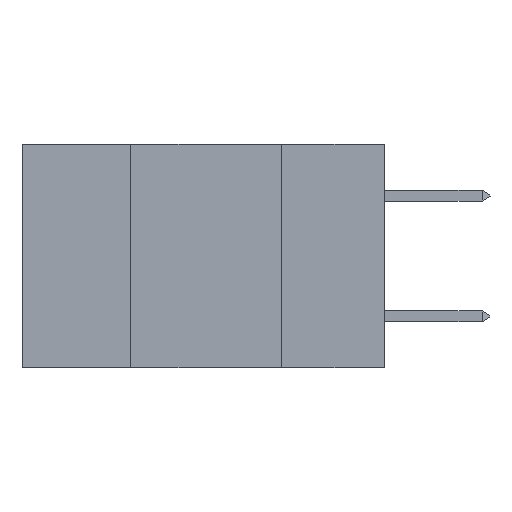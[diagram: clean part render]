
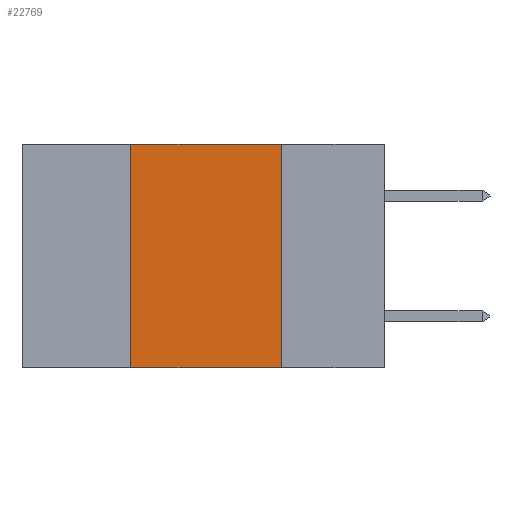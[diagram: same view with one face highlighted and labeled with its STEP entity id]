
A CAD part, left-side view. The second image highlights one B-rep face of the part: STEP entity #22769.
In plain terms, the highlighted planar face has unit normal (-1, 0, 0).
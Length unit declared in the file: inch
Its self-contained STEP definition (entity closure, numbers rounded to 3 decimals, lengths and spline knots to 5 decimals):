
#1746 = ORIENTED_EDGE ( 'NONE', *, *, #6668, .F. ) ;
#2433 = CARTESIAN_POINT ( 'NONE',  ( 0., 0.42, 0. ) ) ;
#4499 = CARTESIAN_POINT ( 'NONE',  ( 0., 0.17, 0. ) ) ;
#6262 = CARTESIAN_POINT ( 'NONE',  ( 0., 0.17, 0. ) ) ;
#6668 = EDGE_CURVE ( 'NONE', #8438, #32411, #27385, .T. ) ;
#8362 = CARTESIAN_POINT ( 'NONE',  ( 0., 0.42, 0. ) ) ;
#8438 = VERTEX_POINT ( 'NONE', #2433 ) ;
#10144 = AXIS2_PLACEMENT_3D ( 'NONE', #35206, #35842, #25653 ) ;
#10730 = CARTESIAN_POINT ( 'NONE',  ( 0., 0.6, 0. ) ) ;
#12917 = ORIENTED_EDGE ( 'NONE', *, *, #26547, .F. ) ;
#15918 = FACE_OUTER_BOUND ( 'NONE', #27540, .T. ) ;
#19678 = LINE ( 'NONE', #6262, #37591 ) ;
#22769 = ADVANCED_FACE ( 'NONE', ( #15918 ), #42349, .F. ) ;
#23365 = VERTEX_POINT ( 'NONE', #29712 ) ;
#23923 = DIRECTION ( 'NONE',  ( 0., -1., 0. ) ) ;
#25653 = DIRECTION ( 'NONE',  ( 0., 0., -1. ) ) ;
#26547 = EDGE_CURVE ( 'NONE', #32411, #34997, #19678, .T. ) ;
#27385 = LINE ( 'NONE', #10730, #27852 ) ;
#27500 = VECTOR ( 'NONE', #41761, 39.37008 ) ;
#27540 = EDGE_LOOP ( 'NONE', ( #12917, #1746, #29695, #37684 ) ) ;
#27852 = VECTOR ( 'NONE', #23923, 39.37008 ) ;
#28569 = EDGE_CURVE ( 'NONE', #23365, #8438, #31727, .T. ) ;
#29695 = ORIENTED_EDGE ( 'NONE', *, *, #28569, .F. ) ;
#29712 = CARTESIAN_POINT ( 'NONE',  ( 0., 0.42, -0.37 ) ) ;
#31727 = LINE ( 'NONE', #8362, #38382 ) ;
#32411 = VERTEX_POINT ( 'NONE', #4499 ) ;
#34997 = VERTEX_POINT ( 'NONE', #39315 ) ;
#35038 = CARTESIAN_POINT ( 'NONE',  ( 0., 0.6, -0.37 ) ) ;
#35206 = CARTESIAN_POINT ( 'NONE',  ( 0., 0.6, 0. ) ) ;
#35712 = DIRECTION ( 'NONE',  ( 0., 0., -1. ) ) ;
#35842 = DIRECTION ( 'NONE',  ( 1., 0., 0. ) ) ;
#37591 = VECTOR ( 'NONE', #35712, 39.37008 ) ;
#37684 = ORIENTED_EDGE ( 'NONE', *, *, #42407, .T. ) ;
#38306 = LINE ( 'NONE', #35038, #27500 ) ;
#38382 = VECTOR ( 'NONE', #41278, 39.37008 ) ;
#39315 = CARTESIAN_POINT ( 'NONE',  ( 0., 0.17, -0.37 ) ) ;
#41278 = DIRECTION ( 'NONE',  ( 0., 0., 1. ) ) ;
#41761 = DIRECTION ( 'NONE',  ( 0., -1., 0. ) ) ;
#42349 = PLANE ( 'NONE',  #10144 ) ;
#42407 = EDGE_CURVE ( 'NONE', #23365, #34997, #38306, .T. ) ;
